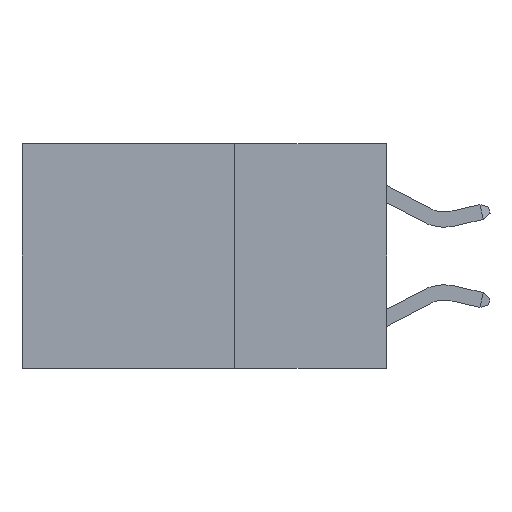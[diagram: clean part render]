
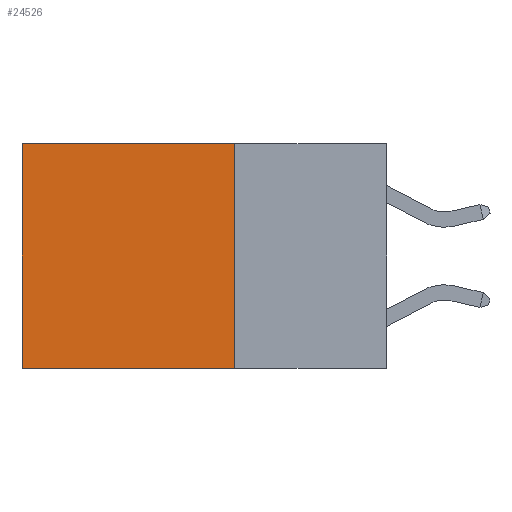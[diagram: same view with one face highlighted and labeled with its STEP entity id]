
A CAD part, left-side view. The second image highlights one B-rep face of the part: STEP entity #24526.
In plain terms, the highlighted planar face has unit normal (-1, 0, 0).
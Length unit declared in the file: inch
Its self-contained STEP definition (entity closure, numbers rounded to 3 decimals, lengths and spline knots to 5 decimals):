
#1528 = VERTEX_POINT ( 'NONE', #16457 ) ;
#1625 = VECTOR ( 'NONE', #27680, 39.37008 ) ;
#1765 = CARTESIAN_POINT ( 'NONE',  ( 0.2625, 0.25, 0. ) ) ;
#1927 = EDGE_CURVE ( 'NONE', #17514, #2238, #2404, .T. ) ;
#2014 = LINE ( 'NONE', #2036, #19998 ) ;
#2036 = CARTESIAN_POINT ( 'NONE',  ( 0.2625, 0.6, 0. ) ) ;
#2238 = VERTEX_POINT ( 'NONE', #26276 ) ;
#2404 = LINE ( 'NONE', #8122, #1625 ) ;
#4247 = DIRECTION ( 'NONE',  ( 0., 0., -1. ) ) ;
#4544 = EDGE_CURVE ( 'NONE', #28801, #17514, #15070, .T. ) ;
#6145 = CARTESIAN_POINT ( 'NONE',  ( 0.2625, 0.25, 0. ) ) ;
#7965 = EDGE_CURVE ( 'NONE', #28801, #1528, #16754, .T. ) ;
#8122 = CARTESIAN_POINT ( 'NONE',  ( 0.2625, 0.25, -0.37 ) ) ;
#9021 = CARTESIAN_POINT ( 'NONE',  ( 0.2625, 0.25, 0. ) ) ;
#10163 = EDGE_LOOP ( 'NONE', ( #21623, #24287, #25059, #24082 ) ) ;
#13292 = CARTESIAN_POINT ( 'NONE',  ( 0.2625, 0.25, 0. ) ) ;
#14021 = PLANE ( 'NONE',  #15456 ) ;
#14326 = VECTOR ( 'NONE', #23356, 39.37008 ) ;
#15070 = LINE ( 'NONE', #6145, #14326 ) ;
#15456 = AXIS2_PLACEMENT_3D ( 'NONE', #1765, #18901, #4247 ) ;
#16336 = EDGE_CURVE ( 'NONE', #1528, #2238, #2014, .T. ) ;
#16457 = CARTESIAN_POINT ( 'NONE',  ( 0.2625, 0.6, 0. ) ) ;
#16713 = DIRECTION ( 'NONE',  ( 0., 0., -1. ) ) ;
#16754 = LINE ( 'NONE', #9021, #29028 ) ;
#17514 = VERTEX_POINT ( 'NONE', #23706 ) ;
#18901 = DIRECTION ( 'NONE',  ( 1., 0., 0. ) ) ;
#19998 = VECTOR ( 'NONE', #16713, 39.37008 ) ;
#21623 = ORIENTED_EDGE ( 'NONE', *, *, #16336, .T. ) ;
#23356 = DIRECTION ( 'NONE',  ( 0., 0., -1. ) ) ;
#23706 = CARTESIAN_POINT ( 'NONE',  ( 0.2625, 0.25, -0.37 ) ) ;
#24082 = ORIENTED_EDGE ( 'NONE', *, *, #7965, .T. ) ;
#24287 = ORIENTED_EDGE ( 'NONE', *, *, #1927, .F. ) ;
#24526 = ADVANCED_FACE ( 'NONE', ( #31280 ), #14021, .F. ) ;
#25059 = ORIENTED_EDGE ( 'NONE', *, *, #4544, .F. ) ;
#26276 = CARTESIAN_POINT ( 'NONE',  ( 0.2625, 0.6, -0.37 ) ) ;
#27680 = DIRECTION ( 'NONE',  ( 0., 1., 0. ) ) ;
#28469 = DIRECTION ( 'NONE',  ( 0., 1., 0. ) ) ;
#28801 = VERTEX_POINT ( 'NONE', #13292 ) ;
#29028 = VECTOR ( 'NONE', #28469, 39.37008 ) ;
#31280 = FACE_OUTER_BOUND ( 'NONE', #10163, .T. ) ;
